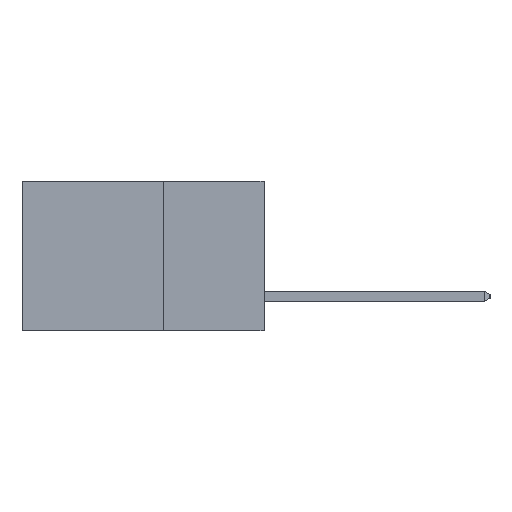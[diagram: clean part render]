
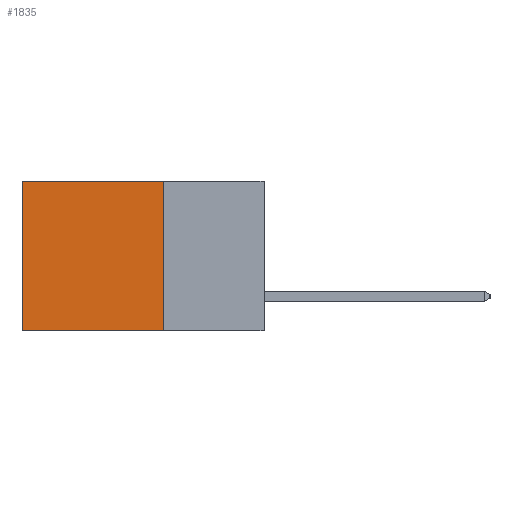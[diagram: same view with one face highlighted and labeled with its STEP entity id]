
A CAD part, left-side view. The second image highlights one B-rep face of the part: STEP entity #1835.
In plain terms, the highlighted planar face has unit normal (-1, 0, 0).
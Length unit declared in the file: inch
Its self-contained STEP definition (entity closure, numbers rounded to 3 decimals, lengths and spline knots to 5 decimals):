
#314 = ORIENTED_EDGE ( 'NONE', *, *, #6074, .T. ) ;
#1159 = FACE_OUTER_BOUND ( 'NONE', #9287, .T. ) ;
#1192 = ORIENTED_EDGE ( 'NONE', *, *, #4010, .T. ) ;
#1835 = ADVANCED_FACE ( 'NONE', ( #1159 ), #17562, .F. ) ;
#2116 = DIRECTION ( 'NONE',  ( 0., 1., 0. ) ) ;
#3055 = ORIENTED_EDGE ( 'NONE', *, *, #16070, .F. ) ;
#3227 = CARTESIAN_POINT ( 'NONE',  ( 0.298, 0.6, -0.37 ) ) ;
#3523 = CARTESIAN_POINT ( 'NONE',  ( 0.298, 0.6, 0. ) ) ;
#3869 = DIRECTION ( 'NONE',  ( 0., 0., -1. ) ) ;
#4010 = EDGE_CURVE ( 'NONE', #24941, #24854, #5283, .T. ) ;
#4022 = VECTOR ( 'NONE', #18281, 39.37008 ) ;
#4158 = ORIENTED_EDGE ( 'NONE', *, *, #14703, .F. ) ;
#5283 = LINE ( 'NONE', #9452, #25348 ) ;
#6074 = EDGE_CURVE ( 'NONE', #14678, #24941, #12065, .T. ) ;
#6165 = CARTESIAN_POINT ( 'NONE',  ( 0.298, 0.25, 0. ) ) ;
#6265 = LINE ( 'NONE', #14693, #16689 ) ;
#7675 = DIRECTION ( 'NONE',  ( 0., 1., 0. ) ) ;
#9287 = EDGE_LOOP ( 'NONE', ( #1192, #3055, #4158, #314 ) ) ;
#9452 = CARTESIAN_POINT ( 'NONE',  ( 0.298, 0.6, 0. ) ) ;
#9578 = CARTESIAN_POINT ( 'NONE',  ( 0.298, 0.25, 0. ) ) ;
#11058 = VERTEX_POINT ( 'NONE', #25654 ) ;
#11411 = VECTOR ( 'NONE', #7675, 39.37008 ) ;
#12065 = LINE ( 'NONE', #9578, #11411 ) ;
#14678 = VERTEX_POINT ( 'NONE', #22215 ) ;
#14693 = CARTESIAN_POINT ( 'NONE',  ( 0.298, 0.25, -0.37 ) ) ;
#14703 = EDGE_CURVE ( 'NONE', #14678, #11058, #26038, .T. ) ;
#15396 = DIRECTION ( 'NONE',  ( 0., 0., -1. ) ) ;
#16070 = EDGE_CURVE ( 'NONE', #11058, #24854, #6265, .T. ) ;
#16689 = VECTOR ( 'NONE', #2116, 39.37008 ) ;
#17562 = PLANE ( 'NONE',  #23002 ) ;
#18281 = DIRECTION ( 'NONE',  ( 0., 0., -1. ) ) ;
#19407 = DIRECTION ( 'NONE',  ( 1., 0., 0. ) ) ;
#22215 = CARTESIAN_POINT ( 'NONE',  ( 0.298, 0.25, 0. ) ) ;
#23002 = AXIS2_PLACEMENT_3D ( 'NONE', #6165, #19407, #15396 ) ;
#24854 = VERTEX_POINT ( 'NONE', #3227 ) ;
#24941 = VERTEX_POINT ( 'NONE', #3523 ) ;
#25348 = VECTOR ( 'NONE', #3869, 39.37008 ) ;
#25654 = CARTESIAN_POINT ( 'NONE',  ( 0.298, 0.25, -0.37 ) ) ;
#26038 = LINE ( 'NONE', #26410, #4022 ) ;
#26410 = CARTESIAN_POINT ( 'NONE',  ( 0.298, 0.25, 0. ) ) ;
